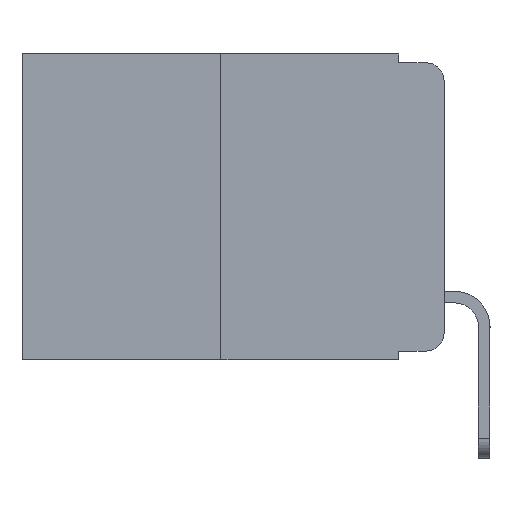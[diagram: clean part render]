
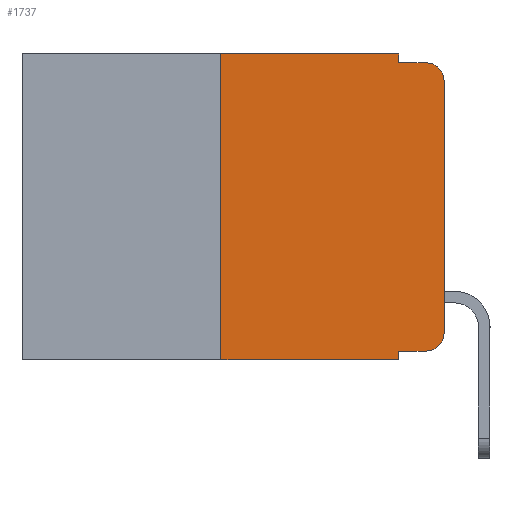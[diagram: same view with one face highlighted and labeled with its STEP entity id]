
A CAD part, left-side view. The second image highlights one B-rep face of the part: STEP entity #1737.
In plain terms, the highlighted planar face has unit normal (-1, 0, 0).
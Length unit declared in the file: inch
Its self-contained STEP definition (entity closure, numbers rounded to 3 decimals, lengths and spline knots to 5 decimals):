
#252 = DIRECTION ( 'NONE',  ( 0., 0., -1. ) ) ;
#349 = CARTESIAN_POINT ( 'NONE',  ( 0., 0.473, -0.343 ) ) ;
#497 = CARTESIAN_POINT ( 'NONE',  ( 0., 0.25, 0. ) ) ;
#568 = CARTESIAN_POINT ( 'NONE',  ( 0., 0.051, -0.333 ) ) ;
#589 = DIRECTION ( 'NONE',  ( -1., 0., 0. ) ) ;
#624 = DIRECTION ( 'NONE',  ( 0., 0., -1. ) ) ;
#727 = CARTESIAN_POINT ( 'NONE',  ( 0., 0.02, -0.01 ) ) ;
#912 = CARTESIAN_POINT ( 'NONE',  ( 0., 0.051, 0. ) ) ;
#1003 = CARTESIAN_POINT ( 'NONE',  ( 0., 0.473, 0. ) ) ;
#1064 = CARTESIAN_POINT ( 'NONE',  ( 0., 0.25, -0.343 ) ) ;
#1168 = DIRECTION ( 'NONE',  ( 0., -1., 0. ) ) ;
#1231 = CARTESIAN_POINT ( 'NONE',  ( 0., 0.051, -0.01 ) ) ;
#1308 = EDGE_CURVE ( 'NONE', #8638, #4963, #9180, .T. ) ;
#1704 = CIRCLE ( 'NONE', #8269, 0.02 ) ;
#1737 = ADVANCED_FACE ( 'NONE', ( #9218 ), #2681, .F. ) ;
#1763 = EDGE_CURVE ( 'NONE', #7865, #6488, #4999, .T. ) ;
#1832 = DIRECTION ( 'NONE',  ( 1., 0., 0. ) ) ;
#1879 = CARTESIAN_POINT ( 'NONE',  ( 0., 0.051, -0.333 ) ) ;
#2183 = ORIENTED_EDGE ( 'NONE', *, *, #8520, .F. ) ;
#2192 = EDGE_CURVE ( 'NONE', #3006, #4749, #6568, .T. ) ;
#2340 = DIRECTION ( 'NONE',  ( 0., 0., -1. ) ) ;
#2671 = DIRECTION ( 'NONE',  ( 0., 0., 1. ) ) ;
#2681 = PLANE ( 'NONE',  #3819 ) ;
#2864 = CARTESIAN_POINT ( 'NONE',  ( 0., 0.02, -0.313 ) ) ;
#2917 = ORIENTED_EDGE ( 'NONE', *, *, #5791, .T. ) ;
#2944 = CARTESIAN_POINT ( 'NONE',  ( 0., 0.051, -0.343 ) ) ;
#3006 = VERTEX_POINT ( 'NONE', #568 ) ;
#3023 = CARTESIAN_POINT ( 'NONE',  ( 0., 0., -0.313 ) ) ;
#3359 = EDGE_LOOP ( 'NONE', ( #6656, #5601, #2183, #4487, #5213, #10451, #2917, #10087, #8504, #5153 ) ) ;
#3461 = LINE ( 'NONE', #7662, #6993 ) ;
#3819 = AXIS2_PLACEMENT_3D ( 'NONE', #8265, #1832, #252 ) ;
#3877 = CARTESIAN_POINT ( 'NONE',  ( 0., 0.02, -0.333 ) ) ;
#4103 = CIRCLE ( 'NONE', #7825, 0.02 ) ;
#4407 = DIRECTION ( 'NONE',  ( 0., -1., 0. ) ) ;
#4487 = ORIENTED_EDGE ( 'NONE', *, *, #10108, .F. ) ;
#4714 = DIRECTION ( 'NONE',  ( 0., 0., -1. ) ) ;
#4729 = EDGE_CURVE ( 'NONE', #6488, #5988, #1704, .T. ) ;
#4749 = VERTEX_POINT ( 'NONE', #3877 ) ;
#4862 = VERTEX_POINT ( 'NONE', #1231 ) ;
#4963 = VERTEX_POINT ( 'NONE', #7818 ) ;
#4999 = LINE ( 'NONE', #5850, #7052 ) ;
#5041 = DIRECTION ( 'NONE',  ( 0., -1., 0. ) ) ;
#5153 = ORIENTED_EDGE ( 'NONE', *, *, #7917, .T. ) ;
#5213 = ORIENTED_EDGE ( 'NONE', *, *, #1308, .F. ) ;
#5601 = ORIENTED_EDGE ( 'NONE', *, *, #4729, .T. ) ;
#5791 = EDGE_CURVE ( 'NONE', #7861, #6299, #9160, .T. ) ;
#5850 = CARTESIAN_POINT ( 'NONE',  ( 0., 0., 0. ) ) ;
#5880 = DIRECTION ( 'NONE',  ( 0., -1., 0. ) ) ;
#5988 = VERTEX_POINT ( 'NONE', #727 ) ;
#6147 = EDGE_CURVE ( 'NONE', #7861, #8638, #8096, .T. ) ;
#6153 = VECTOR ( 'NONE', #5041, 39.37008 ) ;
#6299 = VERTEX_POINT ( 'NONE', #2944 ) ;
#6414 = LINE ( 'NONE', #8896, #7320 ) ;
#6488 = VERTEX_POINT ( 'NONE', #7926 ) ;
#6568 = LINE ( 'NONE', #1879, #6153 ) ;
#6656 = ORIENTED_EDGE ( 'NONE', *, *, #1763, .T. ) ;
#6977 = VECTOR ( 'NONE', #2340, 39.37008 ) ;
#6993 = VECTOR ( 'NONE', #5880, 39.37008 ) ;
#7052 = VECTOR ( 'NONE', #9058, 39.37008 ) ;
#7269 = VECTOR ( 'NONE', #4407, 39.37008 ) ;
#7320 = VECTOR ( 'NONE', #4714, 39.37008 ) ;
#7662 = CARTESIAN_POINT ( 'NONE',  ( 0., 0.051, -0.01 ) ) ;
#7753 = DIRECTION ( 'NONE',  ( 0., 0., -1. ) ) ;
#7818 = CARTESIAN_POINT ( 'NONE',  ( 0., 0.051, 0. ) ) ;
#7825 = AXIS2_PLACEMENT_3D ( 'NONE', #2864, #589, #7753 ) ;
#7840 = CARTESIAN_POINT ( 'NONE',  ( 0., 0.02, -0.03 ) ) ;
#7861 = VERTEX_POINT ( 'NONE', #1064 ) ;
#7865 = VERTEX_POINT ( 'NONE', #3023 ) ;
#7917 = EDGE_CURVE ( 'NONE', #4749, #7865, #4103, .T. ) ;
#7926 = CARTESIAN_POINT ( 'NONE',  ( 0., 0., -0.03 ) ) ;
#7997 = DIRECTION ( 'NONE',  ( -1., 0., 0. ) ) ;
#8096 = LINE ( 'NONE', #9898, #8470 ) ;
#8265 = CARTESIAN_POINT ( 'NONE',  ( 0., 0.473, 0. ) ) ;
#8269 = AXIS2_PLACEMENT_3D ( 'NONE', #7840, #7997, #624 ) ;
#8470 = VECTOR ( 'NONE', #2671, 39.37008 ) ;
#8504 = ORIENTED_EDGE ( 'NONE', *, *, #2192, .T. ) ;
#8520 = EDGE_CURVE ( 'NONE', #4862, #5988, #3461, .T. ) ;
#8638 = VERTEX_POINT ( 'NONE', #497 ) ;
#8782 = EDGE_CURVE ( 'NONE', #3006, #6299, #9622, .T. ) ;
#8896 = CARTESIAN_POINT ( 'NONE',  ( 0., 0.051, 0. ) ) ;
#9058 = DIRECTION ( 'NONE',  ( 0., 0., 1. ) ) ;
#9160 = LINE ( 'NONE', #349, #7269 ) ;
#9180 = LINE ( 'NONE', #1003, #9776 ) ;
#9218 = FACE_OUTER_BOUND ( 'NONE', #3359, .T. ) ;
#9622 = LINE ( 'NONE', #912, #6977 ) ;
#9776 = VECTOR ( 'NONE', #1168, 39.37008 ) ;
#9898 = CARTESIAN_POINT ( 'NONE',  ( 0., 0.25, 0. ) ) ;
#10087 = ORIENTED_EDGE ( 'NONE', *, *, #8782, .F. ) ;
#10108 = EDGE_CURVE ( 'NONE', #4963, #4862, #6414, .T. ) ;
#10451 = ORIENTED_EDGE ( 'NONE', *, *, #6147, .F. ) ;
